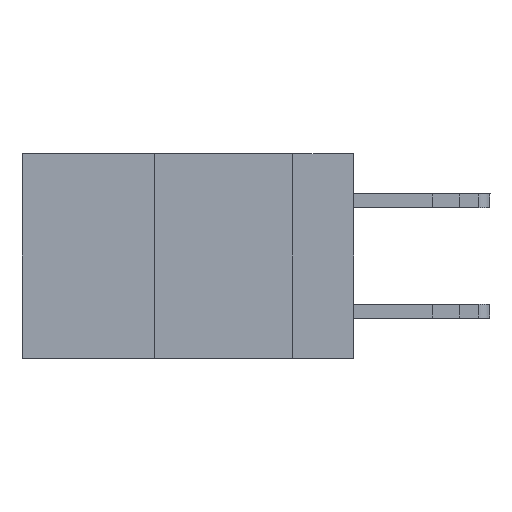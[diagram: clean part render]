
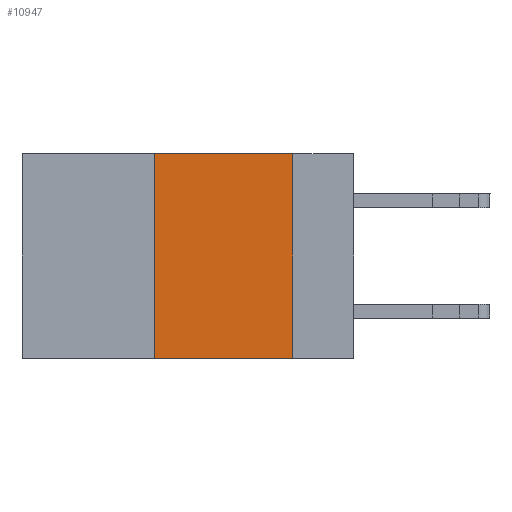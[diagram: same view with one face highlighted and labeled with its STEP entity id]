
A CAD part, left-side view. The second image highlights one B-rep face of the part: STEP entity #10947.
In plain terms, the highlighted planar face has unit normal (-1, 0, 0).
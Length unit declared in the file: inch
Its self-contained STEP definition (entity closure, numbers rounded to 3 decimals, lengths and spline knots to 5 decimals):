
#556 = EDGE_LOOP ( 'NONE', ( #12177, #14081, #3533, #6925 ) ) ;
#1087 = EDGE_CURVE ( 'NONE', #15873, #4464, #4628, .T. ) ;
#1355 = VERTEX_POINT ( 'NONE', #7776 ) ;
#1714 = VECTOR ( 'NONE', #3988, 39.37008 ) ;
#2083 = CARTESIAN_POINT ( 'NONE',  ( 0., 0.6, -0.37 ) ) ;
#3267 = CARTESIAN_POINT ( 'NONE',  ( 0., 0.11, -0.37 ) ) ;
#3533 = ORIENTED_EDGE ( 'NONE', *, *, #1087, .F. ) ;
#3988 = DIRECTION ( 'NONE',  ( 0., 0., -1. ) ) ;
#4464 = VERTEX_POINT ( 'NONE', #11172 ) ;
#4628 = LINE ( 'NONE', #8148, #15478 ) ;
#4852 = LINE ( 'NONE', #16099, #8317 ) ;
#4875 = CARTESIAN_POINT ( 'NONE',  ( 0., 0.36, -0.37 ) ) ;
#5574 = VECTOR ( 'NONE', #11845, 39.37008 ) ;
#6010 = EDGE_CURVE ( 'NONE', #1355, #17562, #7350, .T. ) ;
#6027 = AXIS2_PLACEMENT_3D ( 'NONE', #16298, #17505, #16168 ) ;
#6402 = PLANE ( 'NONE',  #6027 ) ;
#6893 = LINE ( 'NONE', #2083, #5574 ) ;
#6925 = ORIENTED_EDGE ( 'NONE', *, *, #11445, .T. ) ;
#7350 = LINE ( 'NONE', #9610, #1714 ) ;
#7776 = CARTESIAN_POINT ( 'NONE',  ( 0., 0.11, 0. ) ) ;
#7994 = DIRECTION ( 'NONE',  ( 0., 0., 1. ) ) ;
#8148 = CARTESIAN_POINT ( 'NONE',  ( 0., 0.36, 0. ) ) ;
#8317 = VECTOR ( 'NONE', #9099, 39.37008 ) ;
#9099 = DIRECTION ( 'NONE',  ( 0., -1., 0. ) ) ;
#9610 = CARTESIAN_POINT ( 'NONE',  ( 0., 0.11, 0. ) ) ;
#10947 = ADVANCED_FACE ( 'NONE', ( #16467 ), #6402, .F. ) ;
#11172 = CARTESIAN_POINT ( 'NONE',  ( 0., 0.36, 0. ) ) ;
#11445 = EDGE_CURVE ( 'NONE', #15873, #17562, #6893, .T. ) ;
#11845 = DIRECTION ( 'NONE',  ( 0., -1., 0. ) ) ;
#12177 = ORIENTED_EDGE ( 'NONE', *, *, #6010, .F. ) ;
#14081 = ORIENTED_EDGE ( 'NONE', *, *, #14354, .F. ) ;
#14354 = EDGE_CURVE ( 'NONE', #4464, #1355, #4852, .T. ) ;
#15478 = VECTOR ( 'NONE', #7994, 39.37008 ) ;
#15873 = VERTEX_POINT ( 'NONE', #4875 ) ;
#16099 = CARTESIAN_POINT ( 'NONE',  ( 0., 0.6, 0. ) ) ;
#16168 = DIRECTION ( 'NONE',  ( 0., 0., -1. ) ) ;
#16298 = CARTESIAN_POINT ( 'NONE',  ( 0., 0.6, 0. ) ) ;
#16467 = FACE_OUTER_BOUND ( 'NONE', #556, .T. ) ;
#17505 = DIRECTION ( 'NONE',  ( 1., 0., 0. ) ) ;
#17562 = VERTEX_POINT ( 'NONE', #3267 ) ;
